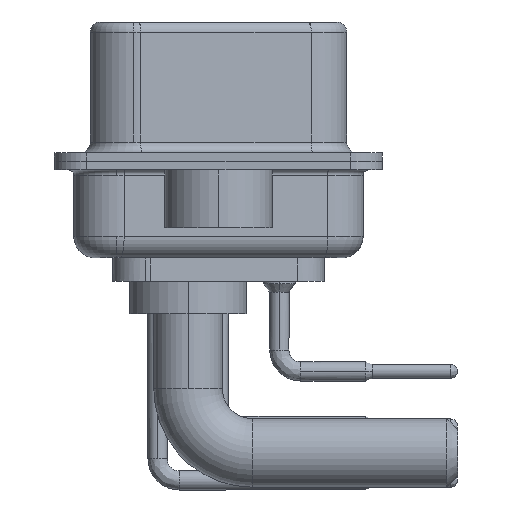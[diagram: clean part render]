
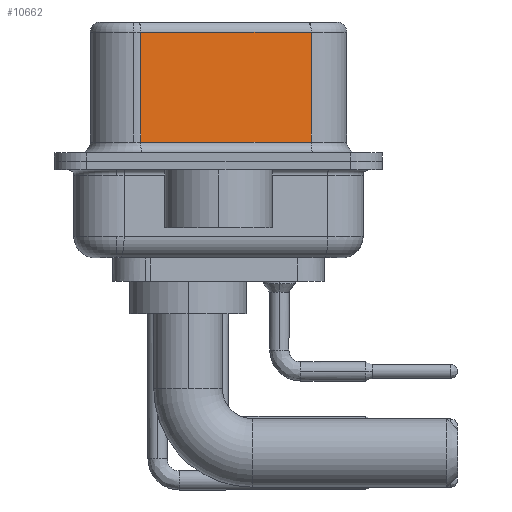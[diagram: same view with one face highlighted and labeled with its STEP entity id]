
A CAD part, left-side view. The second image highlights one B-rep face of the part: STEP entity #10662.
In plain terms, the highlighted planar face has unit normal (-0.985, -0.174, 0).
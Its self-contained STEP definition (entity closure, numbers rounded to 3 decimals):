
#748 = DIRECTION ( 'NONE',  ( 0.174, -0.985, 0. ) ) ;
#1574 = CARTESIAN_POINT ( 'NONE',  ( 5.132, -4.322, 6.02 ) ) ;
#1674 = VERTEX_POINT ( 'NONE', #10972 ) ;
#2292 = ORIENTED_EDGE ( 'NONE', *, *, #9561, .F. ) ;
#3370 = CARTESIAN_POINT ( 'NONE',  ( 3.73, 3.628, 6.52 ) ) ;
#3840 = LINE ( 'NONE', #11472, #24227 ) ;
#6671 = VERTEX_POINT ( 'NONE', #18391 ) ;
#9459 = CARTESIAN_POINT ( 'NONE',  ( 5.132, -4.322, 6.52 ) ) ;
#9519 = EDGE_CURVE ( 'NONE', #6671, #1674, #13940, .T. ) ;
#9561 = EDGE_CURVE ( 'NONE', #19275, #28945, #24007, .T. ) ;
#10653 = VECTOR ( 'NONE', #26623, 1000. ) ;
#10662 = ADVANCED_FACE ( 'NONE', ( #27850 ), #20203, .F. ) ;
#10966 = LINE ( 'NONE', #24654, #20918 ) ;
#10972 = CARTESIAN_POINT ( 'NONE',  ( 3.73, 3.628, 0.9 ) ) ;
#11472 = CARTESIAN_POINT ( 'NONE',  ( 5.132, -4.322, 0.9 ) ) ;
#12410 = DIRECTION ( 'NONE',  ( -0.174, 0.985, 0. ) ) ;
#13940 = LINE ( 'NONE', #3370, #10653 ) ;
#16315 = AXIS2_PLACEMENT_3D ( 'NONE', #9459, #17412, #12410 ) ;
#17412 = DIRECTION ( 'NONE',  ( 0.985, 0.174, 0. ) ) ;
#18391 = CARTESIAN_POINT ( 'NONE',  ( 3.73, 3.628, 6.02 ) ) ;
#19169 = EDGE_LOOP ( 'NONE', ( #2292, #20448, #25661, #29662 ) ) ;
#19275 = VERTEX_POINT ( 'NONE', #1574 ) ;
#19311 = CARTESIAN_POINT ( 'NONE',  ( 5.132, -4.322, 6.52 ) ) ;
#20203 = PLANE ( 'NONE',  #16315 ) ;
#20448 = ORIENTED_EDGE ( 'NONE', *, *, #33731, .T. ) ;
#20659 = VECTOR ( 'NONE', #21752, 1000. ) ;
#20918 = VECTOR ( 'NONE', #26922, 1000. ) ;
#20978 = CARTESIAN_POINT ( 'NONE',  ( 5.132, -4.322, 0.9 ) ) ;
#21752 = DIRECTION ( 'NONE',  ( 0., 0., -1. ) ) ;
#24007 = LINE ( 'NONE', #19311, #20659 ) ;
#24227 = VECTOR ( 'NONE', #748, 1000. ) ;
#24654 = CARTESIAN_POINT ( 'NONE',  ( 5.132, -4.322, 6.02 ) ) ;
#25661 = ORIENTED_EDGE ( 'NONE', *, *, #9519, .T. ) ;
#26623 = DIRECTION ( 'NONE',  ( 0., 0., -1. ) ) ;
#26922 = DIRECTION ( 'NONE',  ( -0.174, 0.985, 0. ) ) ;
#27850 = FACE_OUTER_BOUND ( 'NONE', #19169, .T. ) ;
#28945 = VERTEX_POINT ( 'NONE', #20978 ) ;
#29662 = ORIENTED_EDGE ( 'NONE', *, *, #33796, .T. ) ;
#33731 = EDGE_CURVE ( 'NONE', #19275, #6671, #10966, .T. ) ;
#33796 = EDGE_CURVE ( 'NONE', #1674, #28945, #3840, .T. ) ;
